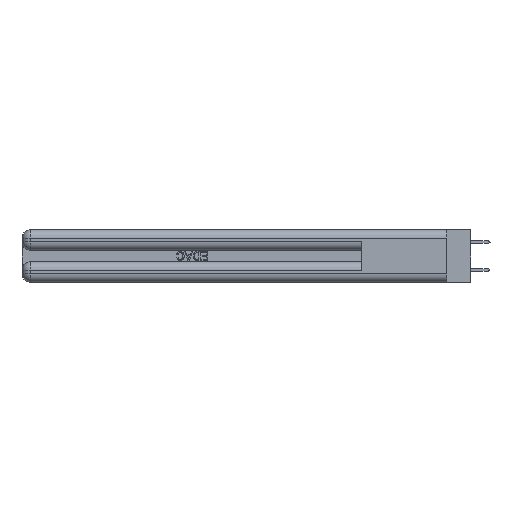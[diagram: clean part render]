
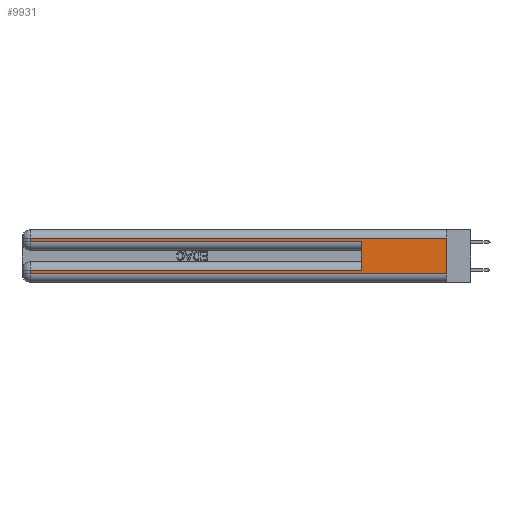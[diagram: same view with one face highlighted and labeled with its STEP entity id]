
A CAD part, left-side view. The second image highlights one B-rep face of the part: STEP entity #9931.
In plain terms, the highlighted planar face has unit normal (-1, 0, 0).
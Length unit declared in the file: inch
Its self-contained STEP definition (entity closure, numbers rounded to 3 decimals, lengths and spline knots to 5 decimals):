
#63 = DIRECTION ( 'NONE',  ( 0., 0., -1. ) ) ;
#346 = CARTESIAN_POINT ( 'NONE',  ( 0., 0., 0.06 ) ) ;
#1232 = VERTEX_POINT ( 'NONE', #5803 ) ;
#1777 = ORIENTED_EDGE ( 'NONE', *, *, #13778, .T. ) ;
#1974 = VERTEX_POINT ( 'NONE', #24799 ) ;
#2446 = VECTOR ( 'NONE', #28300, 39.37008 ) ;
#4303 = LINE ( 'NONE', #32042, #29975 ) ;
#4871 = LINE ( 'NONE', #14867, #2446 ) ;
#5074 = LINE ( 'NONE', #28947, #25112 ) ;
#5803 = CARTESIAN_POINT ( 'NONE',  ( 0., 0., 0.31 ) ) ;
#6132 = CARTESIAN_POINT ( 'NONE',  ( 0., 2.94, 0.06 ) ) ;
#7150 = LINE ( 'NONE', #346, #8654 ) ;
#7454 = AXIS2_PLACEMENT_3D ( 'NONE', #10492, #18232, #63 ) ;
#8069 = ORIENTED_EDGE ( 'NONE', *, *, #8766, .T. ) ;
#8654 = VECTOR ( 'NONE', #31466, 39.37008 ) ;
#8766 = EDGE_CURVE ( 'NONE', #40120, #10358, #4871, .T. ) ;
#8832 = ORIENTED_EDGE ( 'NONE', *, *, #37147, .F. ) ;
#9429 = EDGE_CURVE ( 'NONE', #32700, #10358, #4303, .T. ) ;
#9931 = ADVANCED_FACE ( 'NONE', ( #38673 ), #31638, .F. ) ;
#10358 = VERTEX_POINT ( 'NONE', #34323 ) ;
#10492 = CARTESIAN_POINT ( 'NONE',  ( 0., 0., 0.37 ) ) ;
#10546 = EDGE_CURVE ( 'NONE', #32700, #43069, #28619, .T. ) ;
#13147 = CARTESIAN_POINT ( 'NONE',  ( 0., 0., 0.06 ) ) ;
#13778 = EDGE_CURVE ( 'NONE', #1974, #40120, #20121, .T. ) ;
#14867 = CARTESIAN_POINT ( 'NONE',  ( 0., 0., 0.285 ) ) ;
#15432 = CARTESIAN_POINT ( 'NONE',  ( 0., 0., 0.085 ) ) ;
#15754 = EDGE_CURVE ( 'NONE', #1232, #1974, #22100, .T. ) ;
#17364 = CARTESIAN_POINT ( 'NONE',  ( 0., 2.94, 0.37 ) ) ;
#17851 = VECTOR ( 'NONE', #33994, 39.37008 ) ;
#18087 = CARTESIAN_POINT ( 'NONE',  ( 0., 0.6, 0.085 ) ) ;
#18232 = DIRECTION ( 'NONE',  ( 1., 0., 0. ) ) ;
#18295 = VERTEX_POINT ( 'NONE', #6132 ) ;
#18953 = DIRECTION ( 'NONE',  ( 0., 0., -1. ) ) ;
#19151 = EDGE_CURVE ( 'NONE', #18295, #39242, #7150, .T. ) ;
#19897 = VECTOR ( 'NONE', #26130, 39.37008 ) ;
#19998 = VECTOR ( 'NONE', #42402, 39.37008 ) ;
#20121 = LINE ( 'NONE', #17364, #17851 ) ;
#22100 = LINE ( 'NONE', #32574, #26702 ) ;
#24799 = CARTESIAN_POINT ( 'NONE',  ( 0., 2.94, 0.31 ) ) ;
#25112 = VECTOR ( 'NONE', #18953, 39.37008 ) ;
#26130 = DIRECTION ( 'NONE',  ( 0., 1., 0. ) ) ;
#26702 = VECTOR ( 'NONE', #36191, 39.37008 ) ;
#28300 = DIRECTION ( 'NONE',  ( 0., -1., 0. ) ) ;
#28538 = CARTESIAN_POINT ( 'NONE',  ( 0., 2.94, 0.37 ) ) ;
#28619 = LINE ( 'NONE', #15432, #19897 ) ;
#28947 = CARTESIAN_POINT ( 'NONE',  ( 0., 0., 0.37 ) ) ;
#29975 = VECTOR ( 'NONE', #42719, 39.37008 ) ;
#31466 = DIRECTION ( 'NONE',  ( 0., -1., 0. ) ) ;
#31638 = PLANE ( 'NONE',  #7454 ) ;
#32042 = CARTESIAN_POINT ( 'NONE',  ( 0., 0.6, 0.145 ) ) ;
#32574 = CARTESIAN_POINT ( 'NONE',  ( 0., 0., 0.31 ) ) ;
#32700 = VERTEX_POINT ( 'NONE', #18087 ) ;
#33723 = ORIENTED_EDGE ( 'NONE', *, *, #15754, .T. ) ;
#33994 = DIRECTION ( 'NONE',  ( 0., 0., -1. ) ) ;
#34323 = CARTESIAN_POINT ( 'NONE',  ( 0., 0.6, 0.285 ) ) ;
#34433 = ORIENTED_EDGE ( 'NONE', *, *, #9429, .F. ) ;
#36191 = DIRECTION ( 'NONE',  ( 0., 1., 0. ) ) ;
#36692 = ORIENTED_EDGE ( 'NONE', *, *, #19151, .T. ) ;
#36708 = EDGE_CURVE ( 'NONE', #43069, #18295, #41351, .T. ) ;
#37147 = EDGE_CURVE ( 'NONE', #1232, #39242, #5074, .T. ) ;
#38673 = FACE_OUTER_BOUND ( 'NONE', #40197, .T. ) ;
#39165 = CARTESIAN_POINT ( 'NONE',  ( 0., 2.94, 0.285 ) ) ;
#39242 = VERTEX_POINT ( 'NONE', #13147 ) ;
#39245 = ORIENTED_EDGE ( 'NONE', *, *, #10546, .T. ) ;
#39542 = CARTESIAN_POINT ( 'NONE',  ( 0., 2.94, 0.085 ) ) ;
#40120 = VERTEX_POINT ( 'NONE', #39165 ) ;
#40197 = EDGE_LOOP ( 'NONE', ( #8832, #33723, #1777, #8069, #34433, #39245, #40423, #36692 ) ) ;
#40423 = ORIENTED_EDGE ( 'NONE', *, *, #36708, .T. ) ;
#41351 = LINE ( 'NONE', #28538, #19998 ) ;
#42402 = DIRECTION ( 'NONE',  ( 0., 0., -1. ) ) ;
#42719 = DIRECTION ( 'NONE',  ( 0., 0., 1. ) ) ;
#43069 = VERTEX_POINT ( 'NONE', #39542 ) ;
